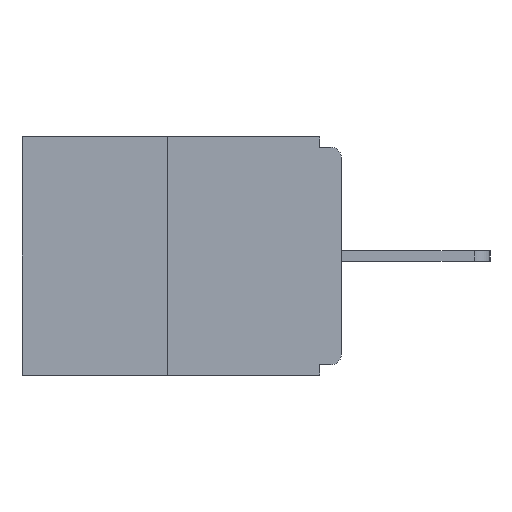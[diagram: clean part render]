
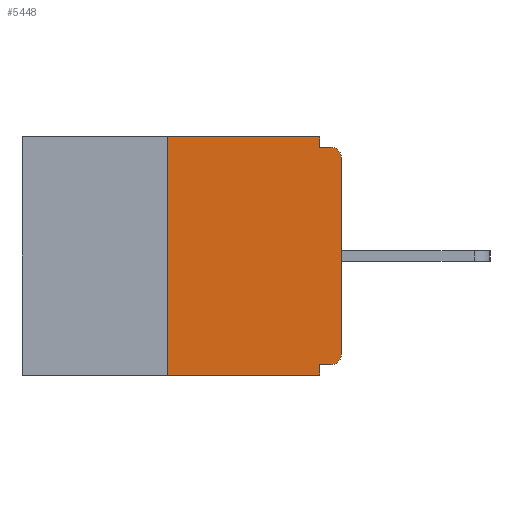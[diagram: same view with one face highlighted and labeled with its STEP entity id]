
A CAD part, left-side view. The second image highlights one B-rep face of the part: STEP entity #5448.
In plain terms, the highlighted planar face has unit normal (-1, 0, 0).
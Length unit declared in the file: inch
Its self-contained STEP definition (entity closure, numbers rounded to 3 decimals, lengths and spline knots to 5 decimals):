
#650 = CIRCLE ( 'NONE', #18228, 0.015 ) ;
#1341 = EDGE_CURVE ( 'NONE', #6621, #18097, #650, .T. ) ;
#1580 = CARTESIAN_POINT ( 'NONE',  ( 0., 0.015, -0.015 ) ) ;
#1631 = ORIENTED_EDGE ( 'NONE', *, *, #11599, .F. ) ;
#2139 = CARTESIAN_POINT ( 'NONE',  ( 0., 0., -0.328 ) ) ;
#2402 = CARTESIAN_POINT ( 'NONE',  ( 0., 0.015, -0.313 ) ) ;
#2691 = EDGE_CURVE ( 'NONE', #11628, #17538, #8504, .T. ) ;
#2702 = LINE ( 'NONE', #15481, #19244 ) ;
#2890 = VERTEX_POINT ( 'NONE', #12847 ) ;
#3231 = EDGE_CURVE ( 'NONE', #9000, #5480, #9772, .T. ) ;
#4358 = CARTESIAN_POINT ( 'NONE',  ( 0., 0.46, 0. ) ) ;
#4413 = VERTEX_POINT ( 'NONE', #19082 ) ;
#4436 = ORIENTED_EDGE ( 'NONE', *, *, #1341, .T. ) ;
#4463 = VERTEX_POINT ( 'NONE', #9723 ) ;
#4966 = ORIENTED_EDGE ( 'NONE', *, *, #7974, .T. ) ;
#5364 = EDGE_CURVE ( 'NONE', #5480, #2890, #20491, .T. ) ;
#5448 = ADVANCED_FACE ( 'NONE', ( #15123 ), #20291, .F. ) ;
#5480 = VERTEX_POINT ( 'NONE', #17148 ) ;
#6621 = VERTEX_POINT ( 'NONE', #13755 ) ;
#6911 = VECTOR ( 'NONE', #10567, 39.37008 ) ;
#7013 = VECTOR ( 'NONE', #14563, 39.37008 ) ;
#7031 = DIRECTION ( 'NONE',  ( 0., 0., 1. ) ) ;
#7275 = DIRECTION ( 'NONE',  ( 0., 0., -1. ) ) ;
#7318 = DIRECTION ( 'NONE',  ( -1., 0., 0. ) ) ;
#7346 = CARTESIAN_POINT ( 'NONE',  ( 0., 0.015, -0.03 ) ) ;
#7380 = CARTESIAN_POINT ( 'NONE',  ( 0., 0.25, 0. ) ) ;
#7649 = DIRECTION ( 'NONE',  ( 0., -1., 0. ) ) ;
#7952 = LINE ( 'NONE', #9893, #16107 ) ;
#7974 = EDGE_CURVE ( 'NONE', #18097, #16563, #21391, .T. ) ;
#8504 = LINE ( 'NONE', #15971, #19982 ) ;
#8928 = DIRECTION ( 'NONE',  ( 0., 1., 0. ) ) ;
#9000 = VERTEX_POINT ( 'NONE', #21216 ) ;
#9183 = CARTESIAN_POINT ( 'NONE',  ( 0., 0., -0.03 ) ) ;
#9630 = DIRECTION ( 'NONE',  ( 0., 0., -1. ) ) ;
#9723 = CARTESIAN_POINT ( 'NONE',  ( 0., 0.031, -0.343 ) ) ;
#9772 = LINE ( 'NONE', #7380, #18392 ) ;
#9893 = CARTESIAN_POINT ( 'NONE',  ( 0., 0.46, -0.343 ) ) ;
#9901 = EDGE_CURVE ( 'NONE', #16563, #17538, #10084, .T. ) ;
#9999 = DIRECTION ( 'NONE',  ( -1., 0., 0. ) ) ;
#10084 = CIRCLE ( 'NONE', #16080, 0.015 ) ;
#10567 = DIRECTION ( 'NONE',  ( 0., -1., 0. ) ) ;
#10672 = CARTESIAN_POINT ( 'NONE',  ( 0., 0.031, -0.015 ) ) ;
#10792 = ORIENTED_EDGE ( 'NONE', *, *, #9901, .T. ) ;
#10978 = ORIENTED_EDGE ( 'NONE', *, *, #5364, .F. ) ;
#11299 = CARTESIAN_POINT ( 'NONE',  ( 0., 0.031, -0.343 ) ) ;
#11599 = EDGE_CURVE ( 'NONE', #2890, #11628, #2702, .T. ) ;
#11628 = VERTEX_POINT ( 'NONE', #10672 ) ;
#12550 = ORIENTED_EDGE ( 'NONE', *, *, #2691, .F. ) ;
#12579 = EDGE_CURVE ( 'NONE', #9000, #4463, #7952, .T. ) ;
#12688 = VECTOR ( 'NONE', #17151, 39.37008 ) ;
#12847 = CARTESIAN_POINT ( 'NONE',  ( 0., 0.031, 0. ) ) ;
#13461 = EDGE_CURVE ( 'NONE', #6621, #4413, #16566, .T. ) ;
#13755 = CARTESIAN_POINT ( 'NONE',  ( 0., 0.015, -0.328 ) ) ;
#14017 = ORIENTED_EDGE ( 'NONE', *, *, #12579, .T. ) ;
#14563 = DIRECTION ( 'NONE',  ( 0., 0., -1. ) ) ;
#14797 = DIRECTION ( 'NONE',  ( 0., -1., 0. ) ) ;
#15123 = FACE_OUTER_BOUND ( 'NONE', #19229, .T. ) ;
#15481 = CARTESIAN_POINT ( 'NONE',  ( 0., 0.031, 0. ) ) ;
#15550 = EDGE_CURVE ( 'NONE', #4413, #4463, #15715, .T. ) ;
#15715 = LINE ( 'NONE', #11299, #7013 ) ;
#15971 = CARTESIAN_POINT ( 'NONE',  ( 0., 0., -0.015 ) ) ;
#16080 = AXIS2_PLACEMENT_3D ( 'NONE', #7346, #7318, #7275 ) ;
#16107 = VECTOR ( 'NONE', #14797, 39.37008 ) ;
#16404 = AXIS2_PLACEMENT_3D ( 'NONE', #20266, #18185, #20867 ) ;
#16519 = ORIENTED_EDGE ( 'NONE', *, *, #13461, .F. ) ;
#16563 = VERTEX_POINT ( 'NONE', #9183 ) ;
#16566 = LINE ( 'NONE', #2139, #18897 ) ;
#17148 = CARTESIAN_POINT ( 'NONE',  ( 0., 0.25, 0. ) ) ;
#17151 = DIRECTION ( 'NONE',  ( 0., 0., 1. ) ) ;
#17356 = CARTESIAN_POINT ( 'NONE',  ( 0., 0., 0. ) ) ;
#17538 = VERTEX_POINT ( 'NONE', #1580 ) ;
#18097 = VERTEX_POINT ( 'NONE', #19541 ) ;
#18185 = DIRECTION ( 'NONE',  ( 1., 0., 0. ) ) ;
#18228 = AXIS2_PLACEMENT_3D ( 'NONE', #2402, #9999, #9630 ) ;
#18392 = VECTOR ( 'NONE', #7031, 39.37008 ) ;
#18855 = ORIENTED_EDGE ( 'NONE', *, *, #15550, .F. ) ;
#18897 = VECTOR ( 'NONE', #8928, 39.37008 ) ;
#19082 = CARTESIAN_POINT ( 'NONE',  ( 0., 0.031, -0.328 ) ) ;
#19229 = EDGE_LOOP ( 'NONE', ( #10978, #20133, #14017, #18855, #16519, #4436, #4966, #10792, #12550, #1631 ) ) ;
#19244 = VECTOR ( 'NONE', #20262, 39.37008 ) ;
#19541 = CARTESIAN_POINT ( 'NONE',  ( 0., 0., -0.313 ) ) ;
#19982 = VECTOR ( 'NONE', #7649, 39.37008 ) ;
#20133 = ORIENTED_EDGE ( 'NONE', *, *, #3231, .F. ) ;
#20262 = DIRECTION ( 'NONE',  ( 0., 0., -1. ) ) ;
#20266 = CARTESIAN_POINT ( 'NONE',  ( 0., 0.46, 0. ) ) ;
#20291 = PLANE ( 'NONE',  #16404 ) ;
#20491 = LINE ( 'NONE', #4358, #6911 ) ;
#20867 = DIRECTION ( 'NONE',  ( 0., 0., -1. ) ) ;
#21216 = CARTESIAN_POINT ( 'NONE',  ( 0., 0.25, -0.343 ) ) ;
#21391 = LINE ( 'NONE', #17356, #12688 ) ;
